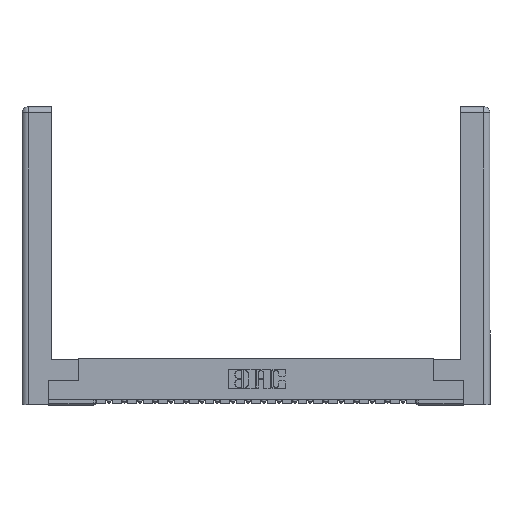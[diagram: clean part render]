
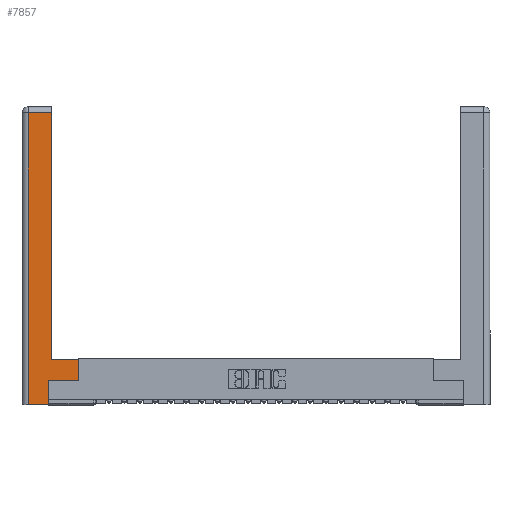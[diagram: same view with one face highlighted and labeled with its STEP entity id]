
A CAD part, top view. The second image highlights one B-rep face of the part: STEP entity #7857.
In plain terms, the highlighted planar face has unit normal (0, 0, 1).
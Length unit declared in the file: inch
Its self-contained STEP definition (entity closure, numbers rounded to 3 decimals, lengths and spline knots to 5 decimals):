
#366 = EDGE_CURVE ( 'NONE', #5555, #20710, #11347, .T. ) ;
#616 = DIRECTION ( 'NONE',  ( 1., 0., 0. ) ) ;
#806 = DIRECTION ( 'NONE',  ( -1., 0., 0. ) ) ;
#1050 = FACE_OUTER_BOUND ( 'NONE', #2836, .T. ) ;
#1173 = CARTESIAN_POINT ( 'NONE',  ( 0., 0., 0. ) ) ;
#1333 = VECTOR ( 'NONE', #24024, 39.37008 ) ;
#2116 = LINE ( 'NONE', #19370, #2304 ) ;
#2163 = EDGE_CURVE ( 'NONE', #18828, #20063, #12295, .T. ) ;
#2304 = VECTOR ( 'NONE', #21186, 39.37008 ) ;
#2349 = VERTEX_POINT ( 'NONE', #15224 ) ;
#2459 = LINE ( 'NONE', #13721, #17593 ) ;
#2836 = EDGE_LOOP ( 'NONE', ( #3399, #4373, #16355, #17902, #9523, #5472, #15624, #15163 ) ) ;
#2959 = CARTESIAN_POINT ( 'NONE',  ( 0.295, 0.45, 0. ) ) ;
#3399 = ORIENTED_EDGE ( 'NONE', *, *, #11220, .T. ) ;
#4373 = ORIENTED_EDGE ( 'NONE', *, *, #16796, .T. ) ;
#5054 = LINE ( 'NONE', #10563, #1333 ) ;
#5472 = ORIENTED_EDGE ( 'NONE', *, *, #12915, .T. ) ;
#5555 = VERTEX_POINT ( 'NONE', #14697 ) ;
#5802 = CARTESIAN_POINT ( 'NONE',  ( 0.265, 0.245, 0. ) ) ;
#6159 = LINE ( 'NONE', #19492, #11682 ) ;
#6880 = EDGE_CURVE ( 'NONE', #12870, #5555, #13614, .T. ) ;
#7276 = CARTESIAN_POINT ( 'NONE',  ( 0.565, 0.245, 0. ) ) ;
#7857 = ADVANCED_FACE ( 'NONE', ( #1050 ), #21482, .F. ) ;
#8329 = CARTESIAN_POINT ( 'NONE',  ( 0.565, 0.45, 0. ) ) ;
#8632 = DIRECTION ( 'NONE',  ( 0., 0., -1. ) ) ;
#9468 = VECTOR ( 'NONE', #806, 39.37008 ) ;
#9523 = ORIENTED_EDGE ( 'NONE', *, *, #2163, .T. ) ;
#9872 = EDGE_CURVE ( 'NONE', #11399, #20446, #2116, .T. ) ;
#10180 = DIRECTION ( 'NONE',  ( 0., 1., 0. ) ) ;
#10563 = CARTESIAN_POINT ( 'NONE',  ( 0.265, 0., 0. ) ) ;
#10703 = DIRECTION ( 'NONE',  ( 0., 1., 0. ) ) ;
#11220 = EDGE_CURVE ( 'NONE', #20710, #2349, #6159, .T. ) ;
#11347 = LINE ( 'NONE', #18816, #14014 ) ;
#11399 = VERTEX_POINT ( 'NONE', #23641 ) ;
#11682 = VECTOR ( 'NONE', #10180, 39.37008 ) ;
#12295 = LINE ( 'NONE', #20004, #18509 ) ;
#12870 = VERTEX_POINT ( 'NONE', #7276 ) ;
#12915 = EDGE_CURVE ( 'NONE', #20063, #12870, #2459, .T. ) ;
#13164 = AXIS2_PLACEMENT_3D ( 'NONE', #1173, #8632, #16097 ) ;
#13313 = DIRECTION ( 'NONE',  ( -1., 0., 0. ) ) ;
#13614 = LINE ( 'NONE', #8329, #23073 ) ;
#13721 = CARTESIAN_POINT ( 'NONE',  ( 0.565, 0.245, 0. ) ) ;
#14014 = VECTOR ( 'NONE', #13313, 39.37008 ) ;
#14697 = CARTESIAN_POINT ( 'NONE',  ( 0.565, 0.45, 0. ) ) ;
#15163 = ORIENTED_EDGE ( 'NONE', *, *, #366, .T. ) ;
#15224 = CARTESIAN_POINT ( 'NONE',  ( 0.295, 2.94, 0. ) ) ;
#15624 = ORIENTED_EDGE ( 'NONE', *, *, #6880, .T. ) ;
#16045 = CARTESIAN_POINT ( 'NONE',  ( 0.265, 0., 0. ) ) ;
#16097 = DIRECTION ( 'NONE',  ( -1., 0., 0. ) ) ;
#16355 = ORIENTED_EDGE ( 'NONE', *, *, #9872, .T. ) ;
#16796 = EDGE_CURVE ( 'NONE', #2349, #11399, #17573, .T. ) ;
#17284 = EDGE_CURVE ( 'NONE', #20446, #18828, #5054, .T. ) ;
#17516 = DIRECTION ( 'NONE',  ( 0., 1., 0. ) ) ;
#17573 = LINE ( 'NONE', #23440, #9468 ) ;
#17593 = VECTOR ( 'NONE', #616, 39.37008 ) ;
#17902 = ORIENTED_EDGE ( 'NONE', *, *, #17284, .T. ) ;
#18509 = VECTOR ( 'NONE', #10703, 39.37008 ) ;
#18816 = CARTESIAN_POINT ( 'NONE',  ( 0.295, 0.45, 0. ) ) ;
#18828 = VERTEX_POINT ( 'NONE', #16045 ) ;
#19370 = CARTESIAN_POINT ( 'NONE',  ( 0.0615, 0., 0. ) ) ;
#19492 = CARTESIAN_POINT ( 'NONE',  ( 0.295, 3., 0. ) ) ;
#20004 = CARTESIAN_POINT ( 'NONE',  ( 0.265, 0.245, 0. ) ) ;
#20063 = VERTEX_POINT ( 'NONE', #5802 ) ;
#20220 = CARTESIAN_POINT ( 'NONE',  ( 0.0615, 0., 0. ) ) ;
#20446 = VERTEX_POINT ( 'NONE', #20220 ) ;
#20710 = VERTEX_POINT ( 'NONE', #2959 ) ;
#21186 = DIRECTION ( 'NONE',  ( 0., -1., 0. ) ) ;
#21482 = PLANE ( 'NONE',  #13164 ) ;
#23073 = VECTOR ( 'NONE', #17516, 39.37008 ) ;
#23440 = CARTESIAN_POINT ( 'NONE',  ( 0.0615, 2.94, 0. ) ) ;
#23641 = CARTESIAN_POINT ( 'NONE',  ( 0.0615, 2.94, 0. ) ) ;
#24024 = DIRECTION ( 'NONE',  ( 1., 0., 0. ) ) ;
